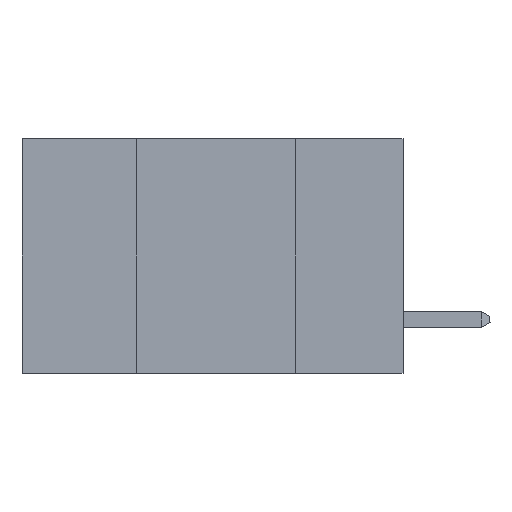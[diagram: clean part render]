
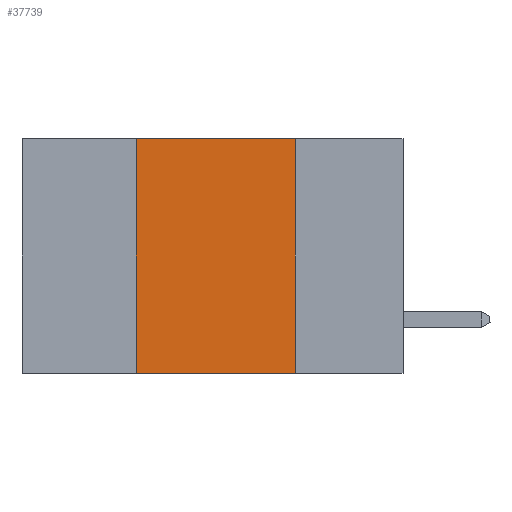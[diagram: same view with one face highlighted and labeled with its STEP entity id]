
A CAD part, left-side view. The second image highlights one B-rep face of the part: STEP entity #37739.
In plain terms, the highlighted planar face has unit normal (-1, 0, 0).
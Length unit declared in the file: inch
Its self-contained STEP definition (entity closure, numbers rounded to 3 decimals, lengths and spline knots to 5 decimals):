
#773 = CARTESIAN_POINT ( 'NONE',  ( 0., 0.6, 0. ) ) ;
#1151 = LINE ( 'NONE', #2027, #12647 ) ;
#2027 = CARTESIAN_POINT ( 'NONE',  ( 0., 0.6, -0.37 ) ) ;
#2934 = EDGE_CURVE ( 'NONE', #30937, #33694, #1151, .T. ) ;
#5023 = FACE_OUTER_BOUND ( 'NONE', #27265, .T. ) ;
#5062 = VECTOR ( 'NONE', #35467, 39.37008 ) ;
#8662 = CARTESIAN_POINT ( 'NONE',  ( 0., 0.42, 0. ) ) ;
#8677 = LINE ( 'NONE', #36546, #28926 ) ;
#9501 = EDGE_CURVE ( 'NONE', #20720, #33694, #36466, .T. ) ;
#12647 = VECTOR ( 'NONE', #29893, 39.37008 ) ;
#14768 = DIRECTION ( 'NONE',  ( 0., 0., 1. ) ) ;
#16421 = DIRECTION ( 'NONE',  ( 0., 0., -1. ) ) ;
#17159 = EDGE_CURVE ( 'NONE', #30937, #24644, #8677, .T. ) ;
#17211 = AXIS2_PLACEMENT_3D ( 'NONE', #32183, #38189, #16421 ) ;
#18575 = CARTESIAN_POINT ( 'NONE',  ( 0., 0.42, -0.37 ) ) ;
#20720 = VERTEX_POINT ( 'NONE', #38536 ) ;
#23011 = VECTOR ( 'NONE', #34800, 39.37008 ) ;
#24644 = VERTEX_POINT ( 'NONE', #8662 ) ;
#24925 = ORIENTED_EDGE ( 'NONE', *, *, #9501, .F. ) ;
#25504 = CARTESIAN_POINT ( 'NONE',  ( 0., 0.17, 0. ) ) ;
#25704 = CARTESIAN_POINT ( 'NONE',  ( 0., 0.17, -0.37 ) ) ;
#27265 = EDGE_LOOP ( 'NONE', ( #24925, #37395, #36068, #36291 ) ) ;
#28926 = VECTOR ( 'NONE', #14768, 39.37008 ) ;
#29893 = DIRECTION ( 'NONE',  ( 0., -1., 0. ) ) ;
#30576 = LINE ( 'NONE', #773, #5062 ) ;
#30937 = VERTEX_POINT ( 'NONE', #18575 ) ;
#32183 = CARTESIAN_POINT ( 'NONE',  ( 0., 0.6, 0. ) ) ;
#33694 = VERTEX_POINT ( 'NONE', #25704 ) ;
#34648 = EDGE_CURVE ( 'NONE', #24644, #20720, #30576, .T. ) ;
#34800 = DIRECTION ( 'NONE',  ( 0., 0., -1. ) ) ;
#34869 = PLANE ( 'NONE',  #17211 ) ;
#35467 = DIRECTION ( 'NONE',  ( 0., -1., 0. ) ) ;
#36068 = ORIENTED_EDGE ( 'NONE', *, *, #17159, .F. ) ;
#36291 = ORIENTED_EDGE ( 'NONE', *, *, #2934, .T. ) ;
#36466 = LINE ( 'NONE', #25504, #23011 ) ;
#36546 = CARTESIAN_POINT ( 'NONE',  ( 0., 0.42, 0. ) ) ;
#37395 = ORIENTED_EDGE ( 'NONE', *, *, #34648, .F. ) ;
#37739 = ADVANCED_FACE ( 'NONE', ( #5023 ), #34869, .F. ) ;
#38189 = DIRECTION ( 'NONE',  ( 1., 0., 0. ) ) ;
#38536 = CARTESIAN_POINT ( 'NONE',  ( 0., 0.17, 0. ) ) ;
